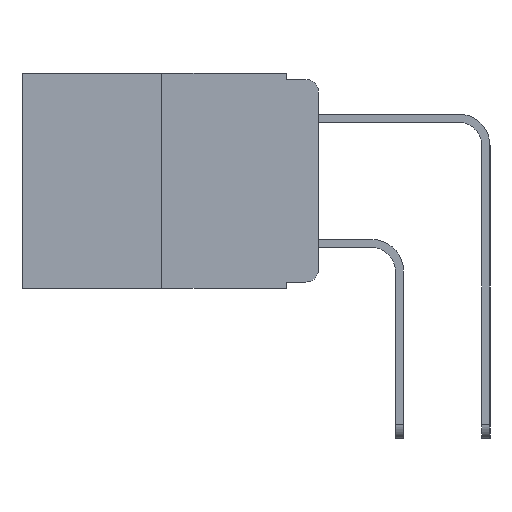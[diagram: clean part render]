
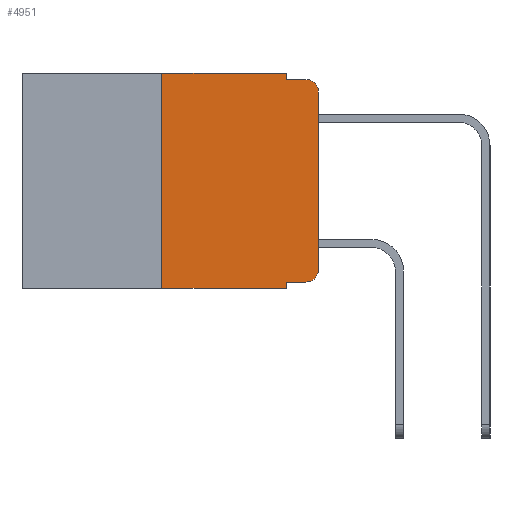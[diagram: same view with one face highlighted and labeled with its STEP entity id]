
A CAD part, left-side view. The second image highlights one B-rep face of the part: STEP entity #4951.
In plain terms, the highlighted planar face has unit normal (-1, 0, 0).
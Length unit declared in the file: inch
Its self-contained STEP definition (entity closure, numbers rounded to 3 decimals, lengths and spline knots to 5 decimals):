
#105 = ORIENTED_EDGE ( 'NONE', *, *, #2166, .F. ) ;
#141 = ORIENTED_EDGE ( 'NONE', *, *, #12285, .F. ) ;
#332 = ORIENTED_EDGE ( 'NONE', *, *, #2095, .F. ) ;
#482 = EDGE_CURVE ( 'NONE', #11026, #13265, #9145, .T. ) ;
#516 = DIRECTION ( 'NONE',  ( 0., 0., -1. ) ) ;
#1333 = VECTOR ( 'NONE', #12219, 39.37008 ) ;
#1457 = CARTESIAN_POINT ( 'NONE',  ( 0., 0.473, 0. ) ) ;
#1493 = CIRCLE ( 'NONE', #2210, 0.02 ) ;
#1520 = DIRECTION ( 'NONE',  ( 0., -1., 0. ) ) ;
#1649 = VECTOR ( 'NONE', #12428, 39.37008 ) ;
#1707 = LINE ( 'NONE', #13204, #1333 ) ;
#1750 = VERTEX_POINT ( 'NONE', #11518 ) ;
#1802 = CARTESIAN_POINT ( 'NONE',  ( 0., 0., 0. ) ) ;
#1840 = CARTESIAN_POINT ( 'NONE',  ( 0., 0.051, -0.01 ) ) ;
#2095 = EDGE_CURVE ( 'NONE', #4429, #9591, #4666, .T. ) ;
#2099 = AXIS2_PLACEMENT_3D ( 'NONE', #6096, #13467, #7229 ) ;
#2166 = EDGE_CURVE ( 'NONE', #7985, #13528, #5826, .T. ) ;
#2178 = CARTESIAN_POINT ( 'NONE',  ( 0., 0.02, -0.313 ) ) ;
#2210 = AXIS2_PLACEMENT_3D ( 'NONE', #2178, #9697, #3304 ) ;
#2217 = DIRECTION ( 'NONE',  ( -1., 0., 0. ) ) ;
#2430 = CARTESIAN_POINT ( 'NONE',  ( 0., 0.051, -0.01 ) ) ;
#2620 = CARTESIAN_POINT ( 'NONE',  ( 0., 0.473, -0.343 ) ) ;
#2787 = CARTESIAN_POINT ( 'NONE',  ( 0., 0.051, -0.343 ) ) ;
#3304 = DIRECTION ( 'NONE',  ( 0., 0., -1. ) ) ;
#3508 = ORIENTED_EDGE ( 'NONE', *, *, #5117, .T. ) ;
#3576 = LINE ( 'NONE', #2620, #11650 ) ;
#4020 = VECTOR ( 'NONE', #12727, 39.37008 ) ;
#4224 = EDGE_LOOP ( 'NONE', ( #11169, #3508, #105, #141, #6666, #332, #9833, #13692, #7942, #10293 ) ) ;
#4390 = VECTOR ( 'NONE', #9009, 39.37008 ) ;
#4429 = VERTEX_POINT ( 'NONE', #6292 ) ;
#4666 = LINE ( 'NONE', #12785, #4020 ) ;
#4811 = EDGE_CURVE ( 'NONE', #11026, #7901, #1707, .T. ) ;
#4923 = VECTOR ( 'NONE', #516, 39.37008 ) ;
#4951 = ADVANCED_FACE ( 'NONE', ( #8249 ), #6138, .F. ) ;
#5117 = EDGE_CURVE ( 'NONE', #9640, #13528, #11511, .T. ) ;
#5826 = LINE ( 'NONE', #2430, #9013 ) ;
#6096 = CARTESIAN_POINT ( 'NONE',  ( 0., 0.473, 0. ) ) ;
#6138 = PLANE ( 'NONE',  #2099 ) ;
#6256 = EDGE_CURVE ( 'NONE', #7901, #8159, #1493, .T. ) ;
#6270 = VECTOR ( 'NONE', #7245, 39.37008 ) ;
#6292 = CARTESIAN_POINT ( 'NONE',  ( 0., 0.25, -0.343 ) ) ;
#6395 = CARTESIAN_POINT ( 'NONE',  ( 0., 0., -0.313 ) ) ;
#6519 = EDGE_CURVE ( 'NONE', #4429, #13265, #3576, .T. ) ;
#6666 = ORIENTED_EDGE ( 'NONE', *, *, #7135, .F. ) ;
#7135 = EDGE_CURVE ( 'NONE', #9591, #1750, #7213, .T. ) ;
#7213 = LINE ( 'NONE', #1457, #4390 ) ;
#7229 = DIRECTION ( 'NONE',  ( 0., 0., -1. ) ) ;
#7245 = DIRECTION ( 'NONE',  ( 0., 0., -1. ) ) ;
#7348 = EDGE_CURVE ( 'NONE', #8159, #9640, #10218, .T. ) ;
#7425 = CARTESIAN_POINT ( 'NONE',  ( 0., 0.02, -0.01 ) ) ;
#7901 = VERTEX_POINT ( 'NONE', #11264 ) ;
#7942 = ORIENTED_EDGE ( 'NONE', *, *, #4811, .T. ) ;
#7985 = VERTEX_POINT ( 'NONE', #1840 ) ;
#8159 = VERTEX_POINT ( 'NONE', #6395 ) ;
#8249 = FACE_OUTER_BOUND ( 'NONE', #4224, .T. ) ;
#8621 = CARTESIAN_POINT ( 'NONE',  ( 0., 0.02, -0.03 ) ) ;
#9009 = DIRECTION ( 'NONE',  ( 0., -1., 0. ) ) ;
#9013 = VECTOR ( 'NONE', #1520, 39.37008 ) ;
#9019 = DIRECTION ( 'NONE',  ( 0., -1., 0. ) ) ;
#9145 = LINE ( 'NONE', #11612, #6270 ) ;
#9591 = VERTEX_POINT ( 'NONE', #10682 ) ;
#9640 = VERTEX_POINT ( 'NONE', #13786 ) ;
#9697 = DIRECTION ( 'NONE',  ( -1., 0., 0. ) ) ;
#9716 = DIRECTION ( 'NONE',  ( 0., 0., -1. ) ) ;
#9833 = ORIENTED_EDGE ( 'NONE', *, *, #6519, .T. ) ;
#10211 = CARTESIAN_POINT ( 'NONE',  ( 0., 0.051, 0. ) ) ;
#10218 = LINE ( 'NONE', #1802, #1649 ) ;
#10293 = ORIENTED_EDGE ( 'NONE', *, *, #6256, .T. ) ;
#10682 = CARTESIAN_POINT ( 'NONE',  ( 0., 0.25, 0. ) ) ;
#11026 = VERTEX_POINT ( 'NONE', #13227 ) ;
#11169 = ORIENTED_EDGE ( 'NONE', *, *, #7348, .T. ) ;
#11264 = CARTESIAN_POINT ( 'NONE',  ( 0., 0.02, -0.333 ) ) ;
#11511 = CIRCLE ( 'NONE', #12036, 0.02 ) ;
#11518 = CARTESIAN_POINT ( 'NONE',  ( 0., 0.051, 0. ) ) ;
#11612 = CARTESIAN_POINT ( 'NONE',  ( 0., 0.051, 0. ) ) ;
#11650 = VECTOR ( 'NONE', #9019, 39.37008 ) ;
#12036 = AXIS2_PLACEMENT_3D ( 'NONE', #8621, #2217, #9716 ) ;
#12219 = DIRECTION ( 'NONE',  ( 0., -1., 0. ) ) ;
#12285 = EDGE_CURVE ( 'NONE', #1750, #7985, #12664, .T. ) ;
#12428 = DIRECTION ( 'NONE',  ( 0., 0., 1. ) ) ;
#12664 = LINE ( 'NONE', #10211, #4923 ) ;
#12727 = DIRECTION ( 'NONE',  ( 0., 0., 1. ) ) ;
#12785 = CARTESIAN_POINT ( 'NONE',  ( 0., 0.25, 0. ) ) ;
#13204 = CARTESIAN_POINT ( 'NONE',  ( 0., 0.051, -0.333 ) ) ;
#13227 = CARTESIAN_POINT ( 'NONE',  ( 0., 0.051, -0.333 ) ) ;
#13265 = VERTEX_POINT ( 'NONE', #2787 ) ;
#13467 = DIRECTION ( 'NONE',  ( 1., 0., 0. ) ) ;
#13528 = VERTEX_POINT ( 'NONE', #7425 ) ;
#13692 = ORIENTED_EDGE ( 'NONE', *, *, #482, .F. ) ;
#13786 = CARTESIAN_POINT ( 'NONE',  ( 0., 0., -0.03 ) ) ;
